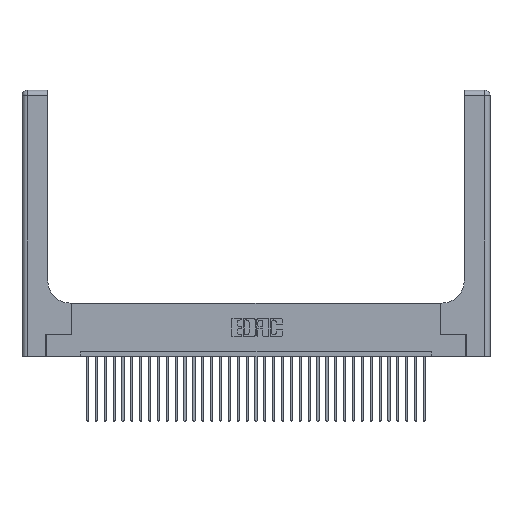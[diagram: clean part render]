
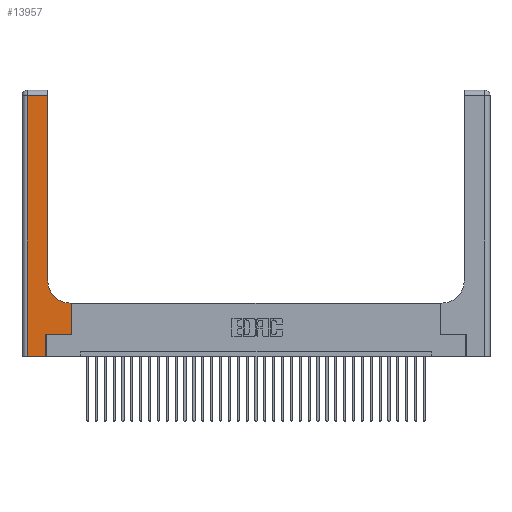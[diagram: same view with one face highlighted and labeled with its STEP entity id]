
A CAD part, top view. The second image highlights one B-rep face of the part: STEP entity #13957.
In plain terms, the highlighted planar face has unit normal (0, 0, 1).
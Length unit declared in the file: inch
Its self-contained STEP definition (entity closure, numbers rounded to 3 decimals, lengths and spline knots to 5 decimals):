
#833 = CIRCLE ( 'NONE', #26272, 0.25 ) ;
#963 = EDGE_CURVE ( 'NONE', #21004, #2546, #34768, .T. ) ;
#1379 = DIRECTION ( 'NONE',  ( 1., 0., 0. ) ) ;
#2343 = EDGE_CURVE ( 'NONE', #34239, #22126, #833, .T. ) ;
#2546 = VERTEX_POINT ( 'NONE', #8146 ) ;
#2667 = VECTOR ( 'NONE', #15566, 39.37008 ) ;
#2907 = DIRECTION ( 'NONE',  ( 0., 0., -1. ) ) ;
#2994 = EDGE_CURVE ( 'NONE', #4293, #33335, #21137, .T. ) ;
#3360 = CARTESIAN_POINT ( 'NONE',  ( 0.06, 2.94, 0.37 ) ) ;
#3742 = ORIENTED_EDGE ( 'NONE', *, *, #32950, .T. ) ;
#3769 = FACE_OUTER_BOUND ( 'NONE', #31939, .T. ) ;
#3835 = EDGE_CURVE ( 'NONE', #23803, #21004, #20599, .T. ) ;
#4293 = VERTEX_POINT ( 'NONE', #22607 ) ;
#4990 = VECTOR ( 'NONE', #27209, 39.37008 ) ;
#6700 = CARTESIAN_POINT ( 'NONE',  ( 0.2915, 3., 0.37 ) ) ;
#8146 = CARTESIAN_POINT ( 'NONE',  ( 0.06, 0., 0.37 ) ) ;
#8803 = ORIENTED_EDGE ( 'NONE', *, *, #10964, .T. ) ;
#9087 = DIRECTION ( 'NONE',  ( -1., 0., 0. ) ) ;
#9329 = ORIENTED_EDGE ( 'NONE', *, *, #3835, .T. ) ;
#9349 = DIRECTION ( 'NONE',  ( 0., 0., -1. ) ) ;
#9391 = DIRECTION ( 'NONE',  ( 0., 1., 0. ) ) ;
#9790 = CARTESIAN_POINT ( 'NONE',  ( 0.2915, 2.94, 0.37 ) ) ;
#9837 = LINE ( 'NONE', #31724, #2667 ) ;
#10034 = VERTEX_POINT ( 'NONE', #28453 ) ;
#10485 = DIRECTION ( 'NONE',  ( -1., 0., 0. ) ) ;
#10805 = EDGE_CURVE ( 'NONE', #33335, #34239, #14182, .T. ) ;
#10964 = EDGE_CURVE ( 'NONE', #22126, #23803, #15030, .T. ) ;
#10992 = CARTESIAN_POINT ( 'NONE',  ( 0.269, 0.25, 0.37 ) ) ;
#11739 = EDGE_CURVE ( 'NONE', #27531, #10034, #20492, .T. ) ;
#13315 = VECTOR ( 'NONE', #9391, 39.37008 ) ;
#13957 = ADVANCED_FACE ( 'NONE', ( #3769 ), #32440, .F. ) ;
#14073 = DIRECTION ( 'NONE',  ( 1., 0., 0. ) ) ;
#14182 = LINE ( 'NONE', #33196, #26042 ) ;
#15030 = LINE ( 'NONE', #6700, #23914 ) ;
#15108 = ORIENTED_EDGE ( 'NONE', *, *, #10805, .T. ) ;
#15517 = DIRECTION ( 'NONE',  ( 0., 1., 0. ) ) ;
#15566 = DIRECTION ( 'NONE',  ( 1., 0., 0. ) ) ;
#16506 = CARTESIAN_POINT ( 'NONE',  ( 0.5415, 0.6, 0.37 ) ) ;
#18953 = ORIENTED_EDGE ( 'NONE', *, *, #21978, .T. ) ;
#20492 = LINE ( 'NONE', #22087, #13315 ) ;
#20599 = LINE ( 'NONE', #31862, #26080 ) ;
#20883 = AXIS2_PLACEMENT_3D ( 'NONE', #29754, #2907, #27238 ) ;
#21004 = VERTEX_POINT ( 'NONE', #3360 ) ;
#21137 = LINE ( 'NONE', #22030, #4990 ) ;
#21978 = EDGE_CURVE ( 'NONE', #2546, #27531, #9837, .T. ) ;
#22030 = CARTESIAN_POINT ( 'NONE',  ( 0.5585, 0.25, 0.37 ) ) ;
#22087 = CARTESIAN_POINT ( 'NONE',  ( 0.269, 0., 0.37 ) ) ;
#22126 = VERTEX_POINT ( 'NONE', #29425 ) ;
#22607 = CARTESIAN_POINT ( 'NONE',  ( 0.5585, 0.25, 0.37 ) ) ;
#22865 = CARTESIAN_POINT ( 'NONE',  ( 0.5415, 0.85, 0.37 ) ) ;
#23803 = VERTEX_POINT ( 'NONE', #9790 ) ;
#23914 = VECTOR ( 'NONE', #15517, 39.37008 ) ;
#25836 = ORIENTED_EDGE ( 'NONE', *, *, #11739, .T. ) ;
#26042 = VECTOR ( 'NONE', #9087, 39.37008 ) ;
#26078 = DIRECTION ( 'NONE',  ( 0., -1., 0. ) ) ;
#26080 = VECTOR ( 'NONE', #10485, 39.37008 ) ;
#26272 = AXIS2_PLACEMENT_3D ( 'NONE', #22865, #9349, #1379 ) ;
#27209 = DIRECTION ( 'NONE',  ( 0., 1., 0. ) ) ;
#27238 = DIRECTION ( 'NONE',  ( -1., 0., 0. ) ) ;
#27531 = VERTEX_POINT ( 'NONE', #32564 ) ;
#27954 = VECTOR ( 'NONE', #26078, 39.37008 ) ;
#28453 = CARTESIAN_POINT ( 'NONE',  ( 0.269, 0.25, 0.37 ) ) ;
#28845 = CARTESIAN_POINT ( 'NONE',  ( 0.5585, 0.6, 0.37 ) ) ;
#29318 = LINE ( 'NONE', #10992, #32245 ) ;
#29425 = CARTESIAN_POINT ( 'NONE',  ( 0.2915, 0.85, 0.37 ) ) ;
#29555 = ORIENTED_EDGE ( 'NONE', *, *, #2994, .T. ) ;
#29754 = CARTESIAN_POINT ( 'NONE',  ( 0., 3., 0.37 ) ) ;
#31724 = CARTESIAN_POINT ( 'NONE',  ( 0., 0., 0.37 ) ) ;
#31862 = CARTESIAN_POINT ( 'NONE',  ( 0., 2.94, 0.37 ) ) ;
#31939 = EDGE_LOOP ( 'NONE', ( #8803, #9329, #34605, #18953, #25836, #3742, #29555, #15108, #34065 ) ) ;
#32245 = VECTOR ( 'NONE', #14073, 39.37008 ) ;
#32440 = PLANE ( 'NONE',  #20883 ) ;
#32564 = CARTESIAN_POINT ( 'NONE',  ( 0.269, 0., 0.37 ) ) ;
#32950 = EDGE_CURVE ( 'NONE', #10034, #4293, #29318, .T. ) ;
#33196 = CARTESIAN_POINT ( 'NONE',  ( 0.2915, 0.6, 0.37 ) ) ;
#33335 = VERTEX_POINT ( 'NONE', #28845 ) ;
#33602 = CARTESIAN_POINT ( 'NONE',  ( 0.06, 3., 0.37 ) ) ;
#34065 = ORIENTED_EDGE ( 'NONE', *, *, #2343, .T. ) ;
#34239 = VERTEX_POINT ( 'NONE', #16506 ) ;
#34605 = ORIENTED_EDGE ( 'NONE', *, *, #963, .T. ) ;
#34768 = LINE ( 'NONE', #33602, #27954 ) ;
